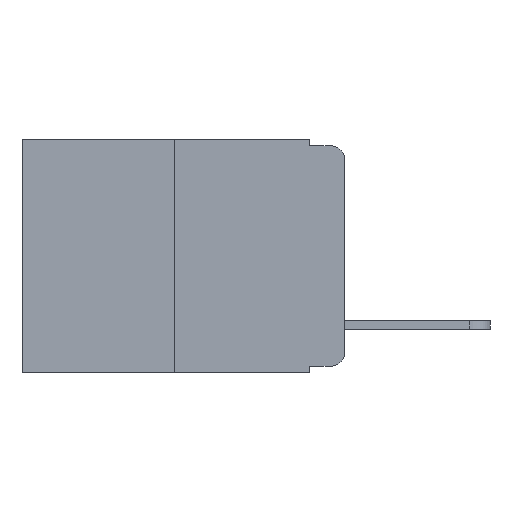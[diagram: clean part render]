
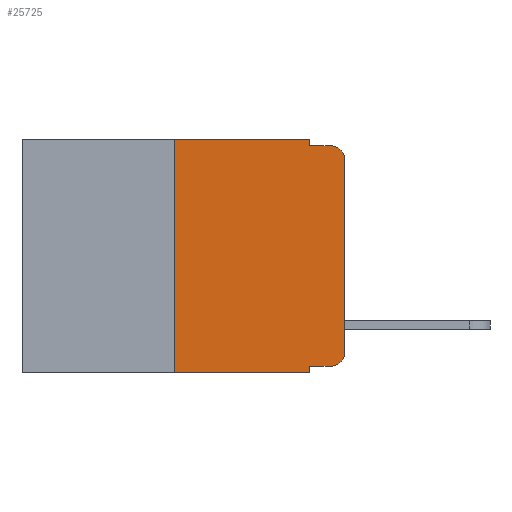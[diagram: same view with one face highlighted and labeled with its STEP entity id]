
A CAD part, left-side view. The second image highlights one B-rep face of the part: STEP entity #25725.
In plain terms, the highlighted planar face has unit normal (-1, 0, 0).
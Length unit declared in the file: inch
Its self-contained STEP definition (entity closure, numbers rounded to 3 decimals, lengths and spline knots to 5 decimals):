
#514 = CIRCLE ( 'NONE', #4378, 0.02 ) ;
#730 = CARTESIAN_POINT ( 'NONE',  ( 0., 0.25, -0.343 ) ) ;
#744 = ORIENTED_EDGE ( 'NONE', *, *, #19025, .T. ) ;
#1219 = ORIENTED_EDGE ( 'NONE', *, *, #10116, .T. ) ;
#2268 = VECTOR ( 'NONE', #23085, 39.37008 ) ;
#2339 = DIRECTION ( 'NONE',  ( 0., -1., 0. ) ) ;
#2419 = CARTESIAN_POINT ( 'NONE',  ( 0., 0.051, -0.01 ) ) ;
#2764 = VERTEX_POINT ( 'NONE', #12796 ) ;
#2908 = LINE ( 'NONE', #7489, #3845 ) ;
#3091 = VERTEX_POINT ( 'NONE', #22120 ) ;
#3235 = LINE ( 'NONE', #24457, #2268 ) ;
#3328 = LINE ( 'NONE', #11695, #14521 ) ;
#3845 = VECTOR ( 'NONE', #19418, 39.37008 ) ;
#4378 = AXIS2_PLACEMENT_3D ( 'NONE', #25234, #17118, #13286 ) ;
#5126 = LINE ( 'NONE', #6072, #15726 ) ;
#6072 = CARTESIAN_POINT ( 'NONE',  ( 0., 0.473, -0.343 ) ) ;
#6195 = PLANE ( 'NONE',  #17850 ) ;
#6253 = ORIENTED_EDGE ( 'NONE', *, *, #20877, .F. ) ;
#6264 = CARTESIAN_POINT ( 'NONE',  ( 0., 0.473, 0. ) ) ;
#6306 = DIRECTION ( 'NONE',  ( 0., 0., -1. ) ) ;
#7164 = CARTESIAN_POINT ( 'NONE',  ( 0., 0.02, -0.313 ) ) ;
#7489 = CARTESIAN_POINT ( 'NONE',  ( 0., 0.25, 0. ) ) ;
#8382 = EDGE_CURVE ( 'NONE', #2764, #21794, #3235, .T. ) ;
#9078 = ORIENTED_EDGE ( 'NONE', *, *, #8382, .F. ) ;
#9293 = VECTOR ( 'NONE', #11601, 39.37008 ) ;
#9812 = EDGE_CURVE ( 'NONE', #24972, #3091, #18921, .T. ) ;
#10116 = EDGE_CURVE ( 'NONE', #17981, #15981, #514, .T. ) ;
#10228 = EDGE_CURVE ( 'NONE', #3091, #15947, #13629, .T. ) ;
#10601 = CARTESIAN_POINT ( 'NONE',  ( 0., 0., -0.03 ) ) ;
#10615 = VERTEX_POINT ( 'NONE', #730 ) ;
#11003 = VECTOR ( 'NONE', #15314, 39.37008 ) ;
#11065 = AXIS2_PLACEMENT_3D ( 'NONE', #7164, #21111, #16557 ) ;
#11096 = ORIENTED_EDGE ( 'NONE', *, *, #13848, .F. ) ;
#11504 = EDGE_LOOP ( 'NONE', ( #744, #1219, #20330, #6253, #9078, #11096, #18123, #20727, #19183, #16630 ) ) ;
#11601 = DIRECTION ( 'NONE',  ( 0., -1., 0. ) ) ;
#11695 = CARTESIAN_POINT ( 'NONE',  ( 0., 0., 0. ) ) ;
#11835 = CARTESIAN_POINT ( 'NONE',  ( 0., 0.051, -0.343 ) ) ;
#12008 = LINE ( 'NONE', #24395, #12630 ) ;
#12630 = VECTOR ( 'NONE', #2339, 39.37008 ) ;
#12796 = CARTESIAN_POINT ( 'NONE',  ( 0., 0.25, 0. ) ) ;
#12932 = VECTOR ( 'NONE', #6306, 39.37008 ) ;
#13055 = EDGE_CURVE ( 'NONE', #24972, #24792, #14785, .T. ) ;
#13153 = VERTEX_POINT ( 'NONE', #2419 ) ;
#13286 = DIRECTION ( 'NONE',  ( 0., 0., -1. ) ) ;
#13629 = CIRCLE ( 'NONE', #11065, 0.02 ) ;
#13848 = EDGE_CURVE ( 'NONE', #10615, #2764, #2908, .T. ) ;
#14212 = DIRECTION ( 'NONE',  ( 1., 0., 0. ) ) ;
#14521 = VECTOR ( 'NONE', #25771, 39.37008 ) ;
#14785 = LINE ( 'NONE', #22007, #12932 ) ;
#15314 = DIRECTION ( 'NONE',  ( 0., 0., -1. ) ) ;
#15726 = VECTOR ( 'NONE', #19999, 39.37008 ) ;
#15947 = VERTEX_POINT ( 'NONE', #18721 ) ;
#15981 = VERTEX_POINT ( 'NONE', #22701 ) ;
#16236 = EDGE_CURVE ( 'NONE', #10615, #24792, #5126, .T. ) ;
#16447 = CARTESIAN_POINT ( 'NONE',  ( 0., 0.051, -0.333 ) ) ;
#16557 = DIRECTION ( 'NONE',  ( 0., 0., -1. ) ) ;
#16630 = ORIENTED_EDGE ( 'NONE', *, *, #10228, .T. ) ;
#17118 = DIRECTION ( 'NONE',  ( -1., 0., 0. ) ) ;
#17850 = AXIS2_PLACEMENT_3D ( 'NONE', #6264, #14212, #23985 ) ;
#17981 = VERTEX_POINT ( 'NONE', #10601 ) ;
#18123 = ORIENTED_EDGE ( 'NONE', *, *, #16236, .T. ) ;
#18721 = CARTESIAN_POINT ( 'NONE',  ( 0., 0., -0.313 ) ) ;
#18921 = LINE ( 'NONE', #23407, #9293 ) ;
#19025 = EDGE_CURVE ( 'NONE', #15947, #17981, #3328, .T. ) ;
#19183 = ORIENTED_EDGE ( 'NONE', *, *, #9812, .T. ) ;
#19418 = DIRECTION ( 'NONE',  ( 0., 0., 1. ) ) ;
#19999 = DIRECTION ( 'NONE',  ( 0., -1., 0. ) ) ;
#20330 = ORIENTED_EDGE ( 'NONE', *, *, #23740, .F. ) ;
#20727 = ORIENTED_EDGE ( 'NONE', *, *, #13055, .F. ) ;
#20877 = EDGE_CURVE ( 'NONE', #21794, #13153, #23435, .T. ) ;
#21111 = DIRECTION ( 'NONE',  ( -1., 0., 0. ) ) ;
#21794 = VERTEX_POINT ( 'NONE', #22290 ) ;
#22007 = CARTESIAN_POINT ( 'NONE',  ( 0., 0.051, 0. ) ) ;
#22120 = CARTESIAN_POINT ( 'NONE',  ( 0., 0.02, -0.333 ) ) ;
#22290 = CARTESIAN_POINT ( 'NONE',  ( 0., 0.051, 0. ) ) ;
#22701 = CARTESIAN_POINT ( 'NONE',  ( 0., 0.02, -0.01 ) ) ;
#23085 = DIRECTION ( 'NONE',  ( 0., -1., 0. ) ) ;
#23407 = CARTESIAN_POINT ( 'NONE',  ( 0., 0.051, -0.333 ) ) ;
#23435 = LINE ( 'NONE', #23531, #11003 ) ;
#23456 = FACE_OUTER_BOUND ( 'NONE', #11504, .T. ) ;
#23531 = CARTESIAN_POINT ( 'NONE',  ( 0., 0.051, 0. ) ) ;
#23740 = EDGE_CURVE ( 'NONE', #13153, #15981, #12008, .T. ) ;
#23985 = DIRECTION ( 'NONE',  ( 0., 0., -1. ) ) ;
#24395 = CARTESIAN_POINT ( 'NONE',  ( 0., 0.051, -0.01 ) ) ;
#24457 = CARTESIAN_POINT ( 'NONE',  ( 0., 0.473, 0. ) ) ;
#24792 = VERTEX_POINT ( 'NONE', #11835 ) ;
#24972 = VERTEX_POINT ( 'NONE', #16447 ) ;
#25234 = CARTESIAN_POINT ( 'NONE',  ( 0., 0.02, -0.03 ) ) ;
#25725 = ADVANCED_FACE ( 'NONE', ( #23456 ), #6195, .F. ) ;
#25771 = DIRECTION ( 'NONE',  ( 0., 0., 1. ) ) ;
